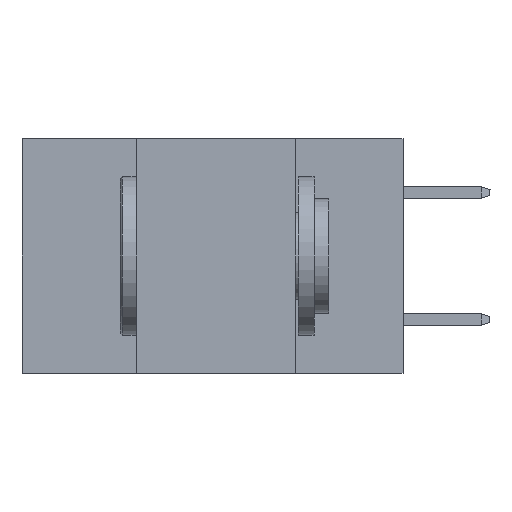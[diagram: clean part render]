
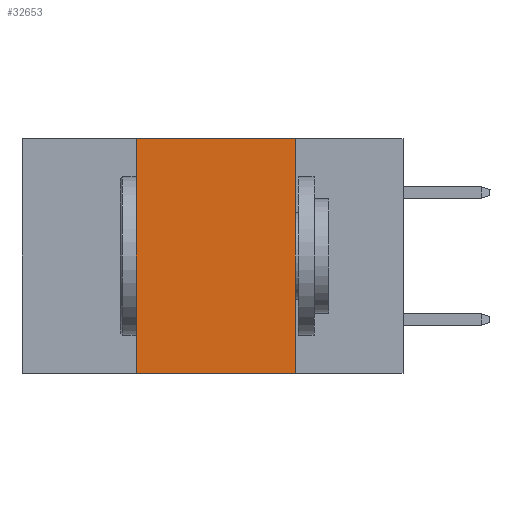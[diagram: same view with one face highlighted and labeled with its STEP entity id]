
A CAD part, left-side view. The second image highlights one B-rep face of the part: STEP entity #32653.
In plain terms, the highlighted planar face has unit normal (-1, 0, 0).
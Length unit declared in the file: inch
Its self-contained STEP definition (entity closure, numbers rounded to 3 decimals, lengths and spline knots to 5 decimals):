
#72 = CARTESIAN_POINT ( 'NONE',  ( 0., 0.6, 0. ) ) ;
#2256 = CARTESIAN_POINT ( 'NONE',  ( 0., 0.17, 0. ) ) ;
#2887 = EDGE_CURVE ( 'NONE', #35457, #23602, #43289, .T. ) ;
#2958 = DIRECTION ( 'NONE',  ( 0., 0., 1. ) ) ;
#4514 = LINE ( 'NONE', #34330, #25654 ) ;
#5374 = CARTESIAN_POINT ( 'NONE',  ( 0., 0.42, -0.37 ) ) ;
#6057 = EDGE_LOOP ( 'NONE', ( #13433, #41134, #14764, #36033 ) ) ;
#6076 = DIRECTION ( 'NONE',  ( 1., 0., 0. ) ) ;
#6439 = DIRECTION ( 'NONE',  ( 0., 0., -1. ) ) ;
#6925 = PLANE ( 'NONE',  #41494 ) ;
#9619 = FACE_OUTER_BOUND ( 'NONE', #6057, .T. ) ;
#9908 = VERTEX_POINT ( 'NONE', #5374 ) ;
#11086 = VECTOR ( 'NONE', #2958, 39.37008 ) ;
#13433 = ORIENTED_EDGE ( 'NONE', *, *, #2887, .F. ) ;
#14764 = ORIENTED_EDGE ( 'NONE', *, *, #16545, .F. ) ;
#16545 = EDGE_CURVE ( 'NONE', #9908, #24905, #42702, .T. ) ;
#18809 = LINE ( 'NONE', #32471, #31456 ) ;
#19090 = EDGE_CURVE ( 'NONE', #24905, #35457, #18809, .T. ) ;
#21279 = CARTESIAN_POINT ( 'NONE',  ( 0., 0.42, 0. ) ) ;
#21725 = EDGE_CURVE ( 'NONE', #9908, #23602, #4514, .T. ) ;
#23602 = VERTEX_POINT ( 'NONE', #32479 ) ;
#24160 = CARTESIAN_POINT ( 'NONE',  ( 0., 0.17, 0. ) ) ;
#24905 = VERTEX_POINT ( 'NONE', #21279 ) ;
#25654 = VECTOR ( 'NONE', #41398, 39.37008 ) ;
#30060 = VECTOR ( 'NONE', #6439, 39.37008 ) ;
#31456 = VECTOR ( 'NONE', #39107, 39.37008 ) ;
#32471 = CARTESIAN_POINT ( 'NONE',  ( 0., 0.6, 0. ) ) ;
#32479 = CARTESIAN_POINT ( 'NONE',  ( 0., 0.17, -0.37 ) ) ;
#32653 = ADVANCED_FACE ( 'NONE', ( #9619 ), #6925, .F. ) ;
#34330 = CARTESIAN_POINT ( 'NONE',  ( 0., 0.6, -0.37 ) ) ;
#35457 = VERTEX_POINT ( 'NONE', #24160 ) ;
#36033 = ORIENTED_EDGE ( 'NONE', *, *, #21725, .T. ) ;
#36940 = DIRECTION ( 'NONE',  ( 0., 0., -1. ) ) ;
#39107 = DIRECTION ( 'NONE',  ( 0., -1., 0. ) ) ;
#41134 = ORIENTED_EDGE ( 'NONE', *, *, #19090, .F. ) ;
#41398 = DIRECTION ( 'NONE',  ( 0., -1., 0. ) ) ;
#41494 = AXIS2_PLACEMENT_3D ( 'NONE', #72, #6076, #36940 ) ;
#42702 = LINE ( 'NONE', #43125, #11086 ) ;
#43125 = CARTESIAN_POINT ( 'NONE',  ( 0., 0.42, 0. ) ) ;
#43289 = LINE ( 'NONE', #2256, #30060 ) ;
